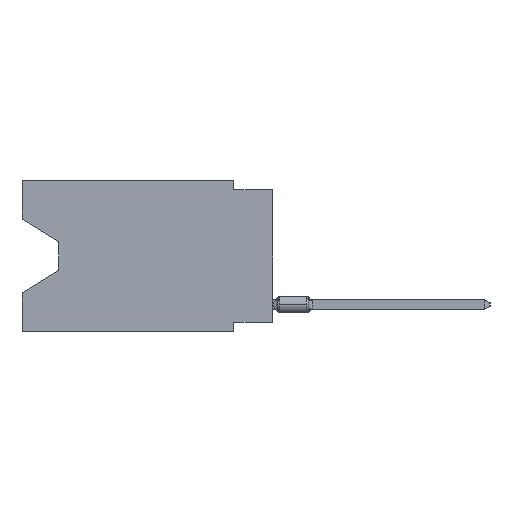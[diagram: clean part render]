
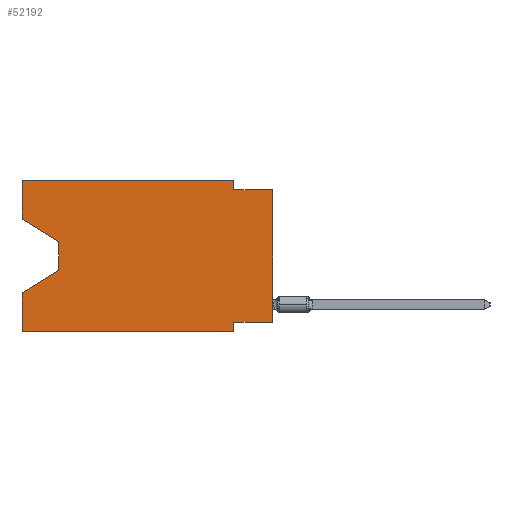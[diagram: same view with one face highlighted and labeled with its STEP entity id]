
A CAD part, left-side view. The second image highlights one B-rep face of the part: STEP entity #52192.
In plain terms, the highlighted planar face has unit normal (-1, 0, 0).
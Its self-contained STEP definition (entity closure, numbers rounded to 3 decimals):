
#164 = DIRECTION ( 'NONE',  ( 0., 0., -1. ) ) ;
#512 = DIRECTION ( 'NONE',  ( 0., 0.855, -0.519 ) ) ;
#571 = CARTESIAN_POINT ( 'NONE',  ( 0., 0., -0.635 ) ) ;
#642 = VECTOR ( 'NONE', #37948, 1000. ) ;
#770 = CARTESIAN_POINT ( 'NONE',  ( 0., 13.97, -4.013 ) ) ;
#2013 = CARTESIAN_POINT ( 'NONE',  ( 0., 2.54, -9.271 ) ) ;
#2941 = CARTESIAN_POINT ( 'NONE',  ( 0., 16.383, 0. ) ) ;
#3421 = CARTESIAN_POINT ( 'NONE',  ( 0., 16.383, -2.546 ) ) ;
#4515 = DIRECTION ( 'NONE',  ( 0., 0., -1. ) ) ;
#4721 = ORIENTED_EDGE ( 'NONE', *, *, #36990, .F. ) ;
#5828 = ORIENTED_EDGE ( 'NONE', *, *, #46155, .F. ) ;
#6115 = CARTESIAN_POINT ( 'NONE',  ( 0., 16.383, 0. ) ) ;
#6477 = ORIENTED_EDGE ( 'NONE', *, *, #64824, .T. ) ;
#6783 = CARTESIAN_POINT ( 'NONE',  ( 0., 0., -9.271 ) ) ;
#7826 = VERTEX_POINT ( 'NONE', #30144 ) ;
#9605 = VERTEX_POINT ( 'NONE', #49588 ) ;
#9728 = DIRECTION ( 'NONE',  ( 0., 0., 1. ) ) ;
#10213 = CARTESIAN_POINT ( 'NONE',  ( 0., 2.54, -9.906 ) ) ;
#10391 = VECTOR ( 'NONE', #164, 1000. ) ;
#11230 = CARTESIAN_POINT ( 'NONE',  ( 0., 13.97, -5.893 ) ) ;
#12303 = EDGE_CURVE ( 'NONE', #32201, #15779, #37633, .T. ) ;
#14275 = CARTESIAN_POINT ( 'NONE',  ( 0., 16.383, -2.546 ) ) ;
#14783 = CARTESIAN_POINT ( 'NONE',  ( 0., 0., -0.635 ) ) ;
#15319 = ORIENTED_EDGE ( 'NONE', *, *, #59233, .F. ) ;
#15779 = VERTEX_POINT ( 'NONE', #49312 ) ;
#18277 = ORIENTED_EDGE ( 'NONE', *, *, #46992, .F. ) ;
#20224 = CARTESIAN_POINT ( 'NONE',  ( 0., 2.54, 0. ) ) ;
#20864 = DIRECTION ( 'NONE',  ( 0., 1., 0. ) ) ;
#21007 = ORIENTED_EDGE ( 'NONE', *, *, #32030, .T. ) ;
#21413 = VERTEX_POINT ( 'NONE', #33253 ) ;
#21766 = ORIENTED_EDGE ( 'NONE', *, *, #30301, .F. ) ;
#21922 = VECTOR ( 'NONE', #46560, 1000. ) ;
#22544 = VERTEX_POINT ( 'NONE', #2013 ) ;
#22589 = VECTOR ( 'NONE', #64550, 1000. ) ;
#22698 = ORIENTED_EDGE ( 'NONE', *, *, #12303, .F. ) ;
#22887 = CARTESIAN_POINT ( 'NONE',  ( 0., 16.383, 0. ) ) ;
#23262 = VECTOR ( 'NONE', #49735, 1000. ) ;
#26237 = LINE ( 'NONE', #770, #30986 ) ;
#27821 = EDGE_CURVE ( 'NONE', #21413, #32291, #48538, .T. ) ;
#27932 = VERTEX_POINT ( 'NONE', #60901 ) ;
#28340 = LINE ( 'NONE', #14275, #23262 ) ;
#28614 = CARTESIAN_POINT ( 'NONE',  ( 0., 16.383, -7.36 ) ) ;
#29166 = LINE ( 'NONE', #34841, #48269 ) ;
#30144 = CARTESIAN_POINT ( 'NONE',  ( 0., 0., -9.271 ) ) ;
#30301 = EDGE_CURVE ( 'NONE', #9605, #58887, #50701, .T. ) ;
#30720 = ORIENTED_EDGE ( 'NONE', *, *, #39481, .F. ) ;
#30986 = VECTOR ( 'NONE', #36623, 1000. ) ;
#31580 = PLANE ( 'NONE',  #59473 ) ;
#32030 = EDGE_CURVE ( 'NONE', #41587, #27932, #26237, .T. ) ;
#32201 = VERTEX_POINT ( 'NONE', #3421 ) ;
#32291 = VERTEX_POINT ( 'NONE', #54297 ) ;
#33253 = CARTESIAN_POINT ( 'NONE',  ( 0., 16.383, -9.906 ) ) ;
#33432 = VECTOR ( 'NONE', #512, 1000. ) ;
#34841 = CARTESIAN_POINT ( 'NONE',  ( 0., 0., 0. ) ) ;
#35346 = LINE ( 'NONE', #10213, #10391 ) ;
#35733 = ORIENTED_EDGE ( 'NONE', *, *, #39341, .T. ) ;
#35940 = DIRECTION ( 'NONE',  ( 0., 0., -1. ) ) ;
#36447 = VECTOR ( 'NONE', #48377, 1000. ) ;
#36623 = DIRECTION ( 'NONE',  ( 0., 0., -1. ) ) ;
#36990 = EDGE_CURVE ( 'NONE', #58887, #43336, #58318, .T. ) ;
#37633 = LINE ( 'NONE', #22887, #642 ) ;
#37948 = DIRECTION ( 'NONE',  ( 0., 0., 1. ) ) ;
#39341 = EDGE_CURVE ( 'NONE', #32201, #41587, #28340, .T. ) ;
#39481 = EDGE_CURVE ( 'NONE', #22544, #32291, #35346, .T. ) ;
#41587 = VERTEX_POINT ( 'NONE', #55708 ) ;
#43336 = VERTEX_POINT ( 'NONE', #571 ) ;
#43469 = LINE ( 'NONE', #2941, #22589 ) ;
#44862 = EDGE_LOOP ( 'NONE', ( #35733, #21007, #59535, #5828, #54606, #30720, #15319, #6477, #4721, #21766, #18277, #22698 ) ) ;
#45981 = DIRECTION ( 'NONE',  ( 1., 0., 0. ) ) ;
#46155 = EDGE_CURVE ( 'NONE', #21413, #49494, #43469, .T. ) ;
#46560 = DIRECTION ( 'NONE',  ( 0., -1., 0. ) ) ;
#46992 = EDGE_CURVE ( 'NONE', #15779, #9605, #64432, .T. ) ;
#48269 = VECTOR ( 'NONE', #9728, 1000. ) ;
#48377 = DIRECTION ( 'NONE',  ( 0., -1., 0. ) ) ;
#48538 = LINE ( 'NONE', #64600, #60536 ) ;
#49312 = CARTESIAN_POINT ( 'NONE',  ( 0., 16.383, 0. ) ) ;
#49381 = EDGE_CURVE ( 'NONE', #27932, #49494, #62140, .T. ) ;
#49494 = VERTEX_POINT ( 'NONE', #28614 ) ;
#49588 = CARTESIAN_POINT ( 'NONE',  ( 0., 2.54, 0. ) ) ;
#49735 = DIRECTION ( 'NONE',  ( 0., -0.855, -0.519 ) ) ;
#50701 = LINE ( 'NONE', #20224, #65094 ) ;
#52192 = ADVANCED_FACE ( 'NONE', ( #57020 ), #31580, .F. ) ;
#52653 = LINE ( 'NONE', #6783, #53100 ) ;
#53100 = VECTOR ( 'NONE', #20864, 1000. ) ;
#54050 = CARTESIAN_POINT ( 'NONE',  ( 0., 16.383, 0. ) ) ;
#54297 = CARTESIAN_POINT ( 'NONE',  ( 0., 2.54, -9.906 ) ) ;
#54606 = ORIENTED_EDGE ( 'NONE', *, *, #27821, .T. ) ;
#55708 = CARTESIAN_POINT ( 'NONE',  ( 0., 13.97, -4.013 ) ) ;
#57020 = FACE_OUTER_BOUND ( 'NONE', #44862, .T. ) ;
#58318 = LINE ( 'NONE', #14783, #21922 ) ;
#58887 = VERTEX_POINT ( 'NONE', #59396 ) ;
#59233 = EDGE_CURVE ( 'NONE', #7826, #22544, #52653, .T. ) ;
#59396 = CARTESIAN_POINT ( 'NONE',  ( 0., 2.54, -0.635 ) ) ;
#59473 = AXIS2_PLACEMENT_3D ( 'NONE', #6115, #45981, #35940 ) ;
#59535 = ORIENTED_EDGE ( 'NONE', *, *, #49381, .T. ) ;
#60536 = VECTOR ( 'NONE', #64272, 1000. ) ;
#60901 = CARTESIAN_POINT ( 'NONE',  ( 0., 13.97, -5.893 ) ) ;
#62140 = LINE ( 'NONE', #11230, #33432 ) ;
#64272 = DIRECTION ( 'NONE',  ( 0., -1., 0. ) ) ;
#64432 = LINE ( 'NONE', #54050, #36447 ) ;
#64550 = DIRECTION ( 'NONE',  ( 0., 0., 1. ) ) ;
#64600 = CARTESIAN_POINT ( 'NONE',  ( 0., 16.383, -9.906 ) ) ;
#64824 = EDGE_CURVE ( 'NONE', #7826, #43336, #29166, .T. ) ;
#65094 = VECTOR ( 'NONE', #4515, 1000. ) ;
